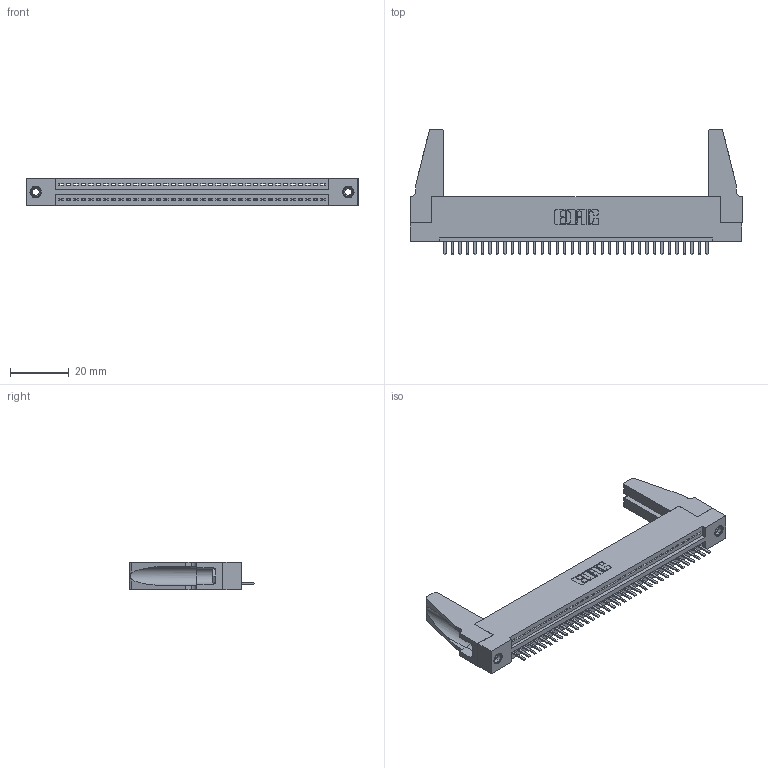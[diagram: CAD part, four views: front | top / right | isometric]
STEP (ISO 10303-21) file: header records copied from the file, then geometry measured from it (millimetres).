
FILE_DESCRIPTION (( 'STEP AP203' ), '1' );
FILE_NAME ('395-036-520-188.STEP', '2019-10-19T20:28:40', ( '' ), ( '' ), 'SwSTEP 2.0', 'SolidWorks 2016', '' );
FILE_SCHEMA (( 'CONFIG_CONTROL_DESIGN' ));
Length unit declared in the file: inch
Products named in the file (5): 345-292-001_345-293-120; 345 Part_Flush Mounting Lugs - 0.156 Dia-TH; 395-036-520-188; 345-220-078_345-220-088; 345-250-001_345-250-001-102
Assembly tree (41 placements, depth 2):
  395-036-520-188
    345 Part_Flush Mounting Lugs - 0.156 Dia-TH
    345-292-001_345-293-120  x36
    345-250-001_345-250-001-102  x2
    345-220-078_345-220-088  x2
Bounding box: 112.67 x 42.55 x 9.4 mm (x, y, z)
Volume: 13801.7 mm3; surface area: 16727.9 mm2
Topology: 41 solids, 41 shells, 2482 faces, 7279 edges, 4746 vertices
Faces by surface type: plane 1664, cylinder 802, cone 12, torus 4
Entity records: 30164 total; most frequent: CARTESIAN_POINT 5226, ORIENTED_EDGE 5144, DIRECTION 4568, EDGE_CURVE 2572, VECTOR 2250, LINE 2250, VERTEX_POINT 1706, AXIS2_PLACEMENT_3D 1159
